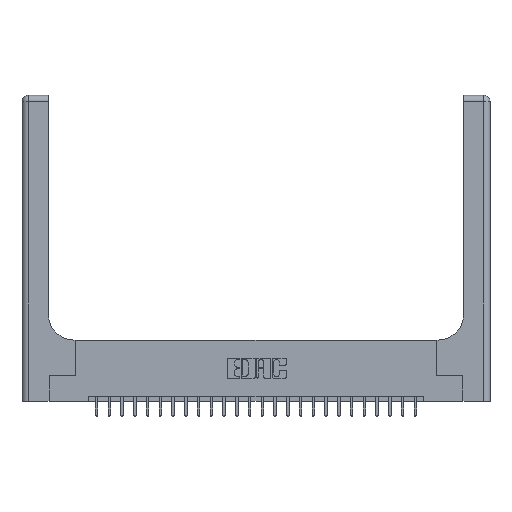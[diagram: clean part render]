
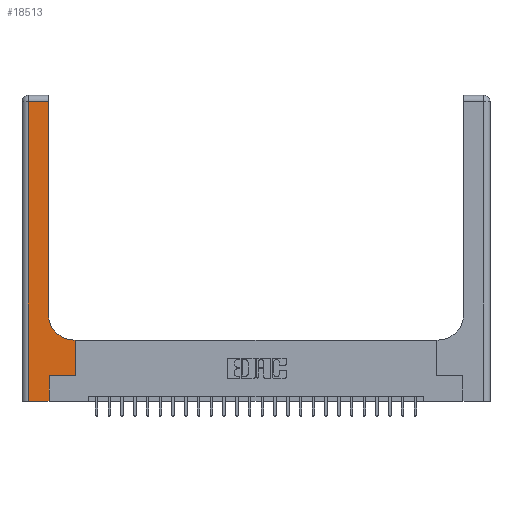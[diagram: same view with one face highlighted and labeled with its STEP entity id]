
A CAD part, top view. The second image highlights one B-rep face of the part: STEP entity #18513.
In plain terms, the highlighted planar face has unit normal (0, 0, 1).
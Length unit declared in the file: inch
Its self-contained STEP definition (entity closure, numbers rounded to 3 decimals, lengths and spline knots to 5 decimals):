
#919 = CARTESIAN_POINT ( 'NONE',  ( 0., 2.94, 0.37 ) ) ;
#998 = EDGE_CURVE ( 'NONE', #4161, #14798, #9259, .T. ) ;
#1591 = DIRECTION ( 'NONE',  ( 0., 0., -1. ) ) ;
#2263 = CARTESIAN_POINT ( 'NONE',  ( 0.265, 0., 0.37 ) ) ;
#3164 = DIRECTION ( 'NONE',  ( 0., -1., 0. ) ) ;
#3434 = VECTOR ( 'NONE', #17559, 39.37008 ) ;
#3760 = DIRECTION ( 'NONE',  ( 0., 1., 0. ) ) ;
#3969 = VERTEX_POINT ( 'NONE', #22045 ) ;
#4113 = VERTEX_POINT ( 'NONE', #5352 ) ;
#4161 = VERTEX_POINT ( 'NONE', #6866 ) ;
#4446 = CARTESIAN_POINT ( 'NONE',  ( 0.265, 0.25, 0.37 ) ) ;
#5352 = CARTESIAN_POINT ( 'NONE',  ( 0.51, 0.6, 0.37 ) ) ;
#5486 = DIRECTION ( 'NONE',  ( -1., 0., 0. ) ) ;
#6039 = EDGE_CURVE ( 'NONE', #17884, #14582, #23255, .T. ) ;
#6792 = LINE ( 'NONE', #11016, #11380 ) ;
#6866 = CARTESIAN_POINT ( 'NONE',  ( 0.528, 0.25, 0.37 ) ) ;
#6980 = ORIENTED_EDGE ( 'NONE', *, *, #15434, .T. ) ;
#7016 = ORIENTED_EDGE ( 'NONE', *, *, #998, .T. ) ;
#7057 = CARTESIAN_POINT ( 'NONE',  ( 0.265, 0., 0.37 ) ) ;
#7285 = DIRECTION ( 'NONE',  ( 0., 0., -1. ) ) ;
#8022 = ORIENTED_EDGE ( 'NONE', *, *, #24235, .T. ) ;
#8323 = LINE ( 'NONE', #21338, #3434 ) ;
#8569 = AXIS2_PLACEMENT_3D ( 'NONE', #22699, #7285, #24486 ) ;
#9259 = LINE ( 'NONE', #21043, #22423 ) ;
#9282 = EDGE_CURVE ( 'NONE', #3969, #18457, #6792, .T. ) ;
#9623 = ORIENTED_EDGE ( 'NONE', *, *, #9282, .T. ) ;
#9754 = LINE ( 'NONE', #919, #18241 ) ;
#9972 = EDGE_CURVE ( 'NONE', #20758, #24592, #17030, .T. ) ;
#11016 = CARTESIAN_POINT ( 'NONE',  ( 0.06, 3., 0.37 ) ) ;
#11223 = CARTESIAN_POINT ( 'NONE',  ( 0.26, 0.6, 0.37 ) ) ;
#11380 = VECTOR ( 'NONE', #3164, 39.37008 ) ;
#11434 = VECTOR ( 'NONE', #19586, 39.37008 ) ;
#11944 = LINE ( 'NONE', #4446, #11434 ) ;
#13816 = VECTOR ( 'NONE', #14554, 39.37008 ) ;
#13823 = VECTOR ( 'NONE', #5486, 39.37008 ) ;
#14006 = ORIENTED_EDGE ( 'NONE', *, *, #23700, .T. ) ;
#14554 = DIRECTION ( 'NONE',  ( 0., 1., 0. ) ) ;
#14582 = VERTEX_POINT ( 'NONE', #14889 ) ;
#14798 = VERTEX_POINT ( 'NONE', #24697 ) ;
#14818 = DIRECTION ( 'NONE',  ( -1., 0., 0. ) ) ;
#14889 = CARTESIAN_POINT ( 'NONE',  ( 0.26, 2.94, 0.37 ) ) ;
#15331 = DIRECTION ( 'NONE',  ( 0., 1., 0. ) ) ;
#15434 = EDGE_CURVE ( 'NONE', #4113, #17884, #23389, .T. ) ;
#15837 = CARTESIAN_POINT ( 'NONE',  ( 0.06, 0., 0.37 ) ) ;
#15902 = DIRECTION ( 'NONE',  ( -1., 0., 0. ) ) ;
#16488 = AXIS2_PLACEMENT_3D ( 'NONE', #22228, #1591, #14818 ) ;
#17030 = LINE ( 'NONE', #7057, #13816 ) ;
#17445 = CARTESIAN_POINT ( 'NONE',  ( 0.26, 3., 0.37 ) ) ;
#17559 = DIRECTION ( 'NONE',  ( 1., 0., 0. ) ) ;
#17707 = VECTOR ( 'NONE', #15331, 39.37008 ) ;
#17884 = VERTEX_POINT ( 'NONE', #22557 ) ;
#17968 = ORIENTED_EDGE ( 'NONE', *, *, #19129, .T. ) ;
#18241 = VECTOR ( 'NONE', #15902, 39.37008 ) ;
#18457 = VERTEX_POINT ( 'NONE', #15837 ) ;
#18513 = ADVANCED_FACE ( 'NONE', ( #20449 ), #18667, .F. ) ;
#18667 = PLANE ( 'NONE',  #16488 ) ;
#19129 = EDGE_CURVE ( 'NONE', #14582, #3969, #9754, .T. ) ;
#19586 = DIRECTION ( 'NONE',  ( 1., 0., 0. ) ) ;
#19672 = CARTESIAN_POINT ( 'NONE',  ( 0.265, 0.25, 0.37 ) ) ;
#20449 = FACE_OUTER_BOUND ( 'NONE', #21886, .T. ) ;
#20476 = ORIENTED_EDGE ( 'NONE', *, *, #9972, .T. ) ;
#20758 = VERTEX_POINT ( 'NONE', #2263 ) ;
#21043 = CARTESIAN_POINT ( 'NONE',  ( 0.528, 0.25, 0.37 ) ) ;
#21338 = CARTESIAN_POINT ( 'NONE',  ( 0., 0., 0.37 ) ) ;
#21886 = EDGE_LOOP ( 'NONE', ( #23156, #17968, #9623, #24300, #20476, #8022, #7016, #14006, #6980 ) ) ;
#22045 = CARTESIAN_POINT ( 'NONE',  ( 0.06, 2.94, 0.37 ) ) ;
#22228 = CARTESIAN_POINT ( 'NONE',  ( 0., 3., 0.37 ) ) ;
#22403 = LINE ( 'NONE', #11223, #13823 ) ;
#22423 = VECTOR ( 'NONE', #3760, 39.37008 ) ;
#22557 = CARTESIAN_POINT ( 'NONE',  ( 0.26, 0.85, 0.37 ) ) ;
#22699 = CARTESIAN_POINT ( 'NONE',  ( 0.51, 0.85, 0.37 ) ) ;
#22946 = EDGE_CURVE ( 'NONE', #18457, #20758, #8323, .T. ) ;
#23156 = ORIENTED_EDGE ( 'NONE', *, *, #6039, .T. ) ;
#23255 = LINE ( 'NONE', #17445, #17707 ) ;
#23389 = CIRCLE ( 'NONE', #8569, 0.25 ) ;
#23700 = EDGE_CURVE ( 'NONE', #14798, #4113, #22403, .T. ) ;
#24235 = EDGE_CURVE ( 'NONE', #24592, #4161, #11944, .T. ) ;
#24300 = ORIENTED_EDGE ( 'NONE', *, *, #22946, .T. ) ;
#24486 = DIRECTION ( 'NONE',  ( 1., 0., 0. ) ) ;
#24592 = VERTEX_POINT ( 'NONE', #19672 ) ;
#24697 = CARTESIAN_POINT ( 'NONE',  ( 0.528, 0.6, 0.37 ) ) ;
